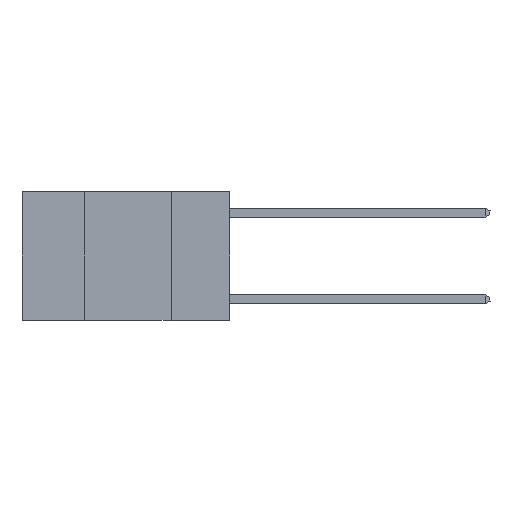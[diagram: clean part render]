
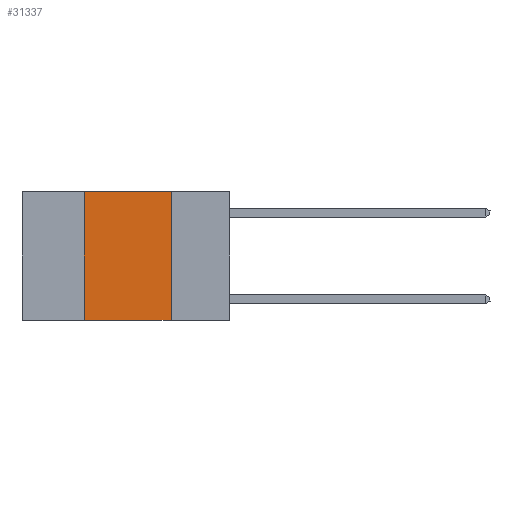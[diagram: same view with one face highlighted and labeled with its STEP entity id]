
A CAD part, left-side view. The second image highlights one B-rep face of the part: STEP entity #31337.
In plain terms, the highlighted planar face has unit normal (-1, 0, 0).
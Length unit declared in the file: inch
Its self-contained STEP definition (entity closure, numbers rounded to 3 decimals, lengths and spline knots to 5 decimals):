
#719 = DIRECTION ( 'NONE',  ( 0., -1., 0. ) ) ;
#1905 = ORIENTED_EDGE ( 'NONE', *, *, #9695, .F. ) ;
#2856 = PLANE ( 'NONE',  #3686 ) ;
#2960 = DIRECTION ( 'NONE',  ( 1., 0., 0. ) ) ;
#3545 = ORIENTED_EDGE ( 'NONE', *, *, #14424, .F. ) ;
#3609 = CARTESIAN_POINT ( 'NONE',  ( 0., 0.17, -0.37 ) ) ;
#3686 = AXIS2_PLACEMENT_3D ( 'NONE', #28333, #2960, #20933 ) ;
#4123 = VERTEX_POINT ( 'NONE', #13708 ) ;
#4704 = VERTEX_POINT ( 'NONE', #10564 ) ;
#4919 = DIRECTION ( 'NONE',  ( 0., 0., 1. ) ) ;
#5143 = VERTEX_POINT ( 'NONE', #22152 ) ;
#5165 = ORIENTED_EDGE ( 'NONE', *, *, #18517, .T. ) ;
#5648 = VECTOR ( 'NONE', #9082, 39.37008 ) ;
#6464 = LINE ( 'NONE', #19214, #5648 ) ;
#8588 = EDGE_CURVE ( 'NONE', #5143, #9081, #14128, .T. ) ;
#9081 = VERTEX_POINT ( 'NONE', #3609 ) ;
#9082 = DIRECTION ( 'NONE',  ( 0., -1., 0. ) ) ;
#9695 = EDGE_CURVE ( 'NONE', #4123, #5143, #15256, .T. ) ;
#10171 = CARTESIAN_POINT ( 'NONE',  ( 0., 0.42, 0. ) ) ;
#10564 = CARTESIAN_POINT ( 'NONE',  ( 0., 0.42, -0.37 ) ) ;
#13330 = VECTOR ( 'NONE', #24722, 39.37008 ) ;
#13708 = CARTESIAN_POINT ( 'NONE',  ( 0., 0.42, 0. ) ) ;
#14128 = LINE ( 'NONE', #27129, #13330 ) ;
#14424 = EDGE_CURVE ( 'NONE', #4704, #4123, #25814, .T. ) ;
#14453 = VECTOR ( 'NONE', #719, 39.37008 ) ;
#14843 = ORIENTED_EDGE ( 'NONE', *, *, #8588, .F. ) ;
#15193 = EDGE_LOOP ( 'NONE', ( #14843, #1905, #3545, #5165 ) ) ;
#15256 = LINE ( 'NONE', #21289, #14453 ) ;
#18517 = EDGE_CURVE ( 'NONE', #4704, #9081, #6464, .T. ) ;
#19214 = CARTESIAN_POINT ( 'NONE',  ( 0., 0.6, -0.37 ) ) ;
#20933 = DIRECTION ( 'NONE',  ( 0., 0., -1. ) ) ;
#21289 = CARTESIAN_POINT ( 'NONE',  ( 0., 0.6, 0. ) ) ;
#22152 = CARTESIAN_POINT ( 'NONE',  ( 0., 0.17, 0. ) ) ;
#23654 = FACE_OUTER_BOUND ( 'NONE', #15193, .T. ) ;
#24722 = DIRECTION ( 'NONE',  ( 0., 0., -1. ) ) ;
#25814 = LINE ( 'NONE', #10171, #32473 ) ;
#27129 = CARTESIAN_POINT ( 'NONE',  ( 0., 0.17, 0. ) ) ;
#28333 = CARTESIAN_POINT ( 'NONE',  ( 0., 0.6, 0. ) ) ;
#31337 = ADVANCED_FACE ( 'NONE', ( #23654 ), #2856, .F. ) ;
#32473 = VECTOR ( 'NONE', #4919, 39.37008 ) ;
